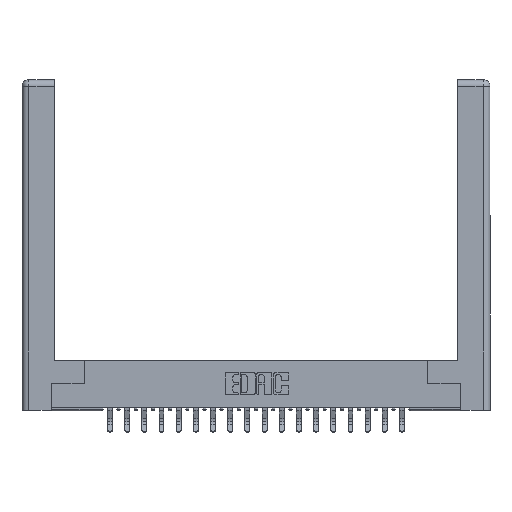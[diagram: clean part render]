
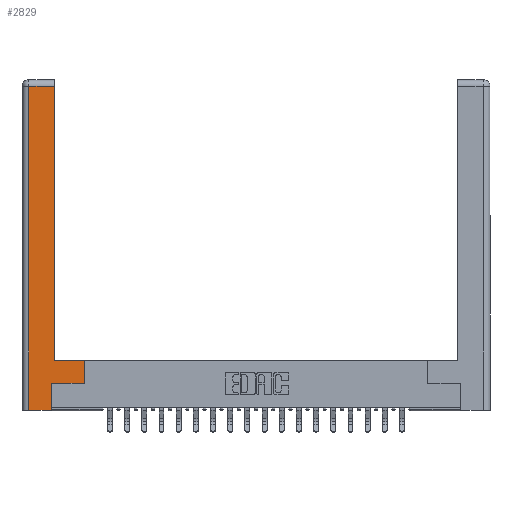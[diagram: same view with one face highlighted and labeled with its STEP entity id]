
A CAD part, top view. The second image highlights one B-rep face of the part: STEP entity #2829.
In plain terms, the highlighted planar face has unit normal (0, 0, 1).
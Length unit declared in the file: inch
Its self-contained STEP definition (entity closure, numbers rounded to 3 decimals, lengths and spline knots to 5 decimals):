
#114 = EDGE_CURVE ( 'NONE', #10199, #15605, #15759, .T. ) ;
#343 = VERTEX_POINT ( 'NONE', #11007 ) ;
#476 = ORIENTED_EDGE ( 'NONE', *, *, #8316, .T. ) ;
#874 = VERTEX_POINT ( 'NONE', #24880 ) ;
#950 = FACE_OUTER_BOUND ( 'NONE', #5604, .T. ) ;
#991 = EDGE_CURVE ( 'NONE', #9284, #343, #18439, .T. ) ;
#1299 = DIRECTION ( 'NONE',  ( 0., 0., -1. ) ) ;
#1379 = CARTESIAN_POINT ( 'NONE',  ( 0., 0., 0. ) ) ;
#2542 = VECTOR ( 'NONE', #3873, 39.37008 ) ;
#2829 = ADVANCED_FACE ( 'NONE', ( #950 ), #22866, .F. ) ;
#3343 = CARTESIAN_POINT ( 'NONE',  ( 0.0615, 2.94, 0. ) ) ;
#3873 = DIRECTION ( 'NONE',  ( 0., 1., 0. ) ) ;
#4245 = DIRECTION ( 'NONE',  ( -1., 0., 0. ) ) ;
#4337 = VECTOR ( 'NONE', #21157, 39.37008 ) ;
#5604 = EDGE_LOOP ( 'NONE', ( #15982, #12240, #10795, #15543, #21265, #24554, #12148, #476 ) ) ;
#5659 = CARTESIAN_POINT ( 'NONE',  ( 0.265, 0., 0. ) ) ;
#5942 = EDGE_CURVE ( 'NONE', #15605, #12000, #15135, .T. ) ;
#6504 = DIRECTION ( 'NONE',  ( 0., -1., 0. ) ) ;
#6518 = EDGE_CURVE ( 'NONE', #7420, #9284, #14197, .T. ) ;
#6595 = LINE ( 'NONE', #22156, #20890 ) ;
#6695 = AXIS2_PLACEMENT_3D ( 'NONE', #1379, #1299, #22707 ) ;
#6805 = CARTESIAN_POINT ( 'NONE',  ( 0.565, 0.245, 0. ) ) ;
#7385 = LINE ( 'NONE', #15557, #4337 ) ;
#7420 = VERTEX_POINT ( 'NONE', #15808 ) ;
#7740 = LINE ( 'NONE', #23475, #2542 ) ;
#8316 = EDGE_CURVE ( 'NONE', #343, #10199, #7385, .T. ) ;
#8689 = DIRECTION ( 'NONE',  ( 1., 0., 0. ) ) ;
#9004 = VECTOR ( 'NONE', #17351, 39.37008 ) ;
#9284 = VERTEX_POINT ( 'NONE', #11108 ) ;
#9619 = CARTESIAN_POINT ( 'NONE',  ( 0.565, 0.45, 0. ) ) ;
#9972 = VECTOR ( 'NONE', #4245, 39.37008 ) ;
#10199 = VERTEX_POINT ( 'NONE', #23012 ) ;
#10268 = CARTESIAN_POINT ( 'NONE',  ( 0.295, 3., 0. ) ) ;
#10795 = ORIENTED_EDGE ( 'NONE', *, *, #22169, .T. ) ;
#11007 = CARTESIAN_POINT ( 'NONE',  ( 0.565, 0.45, 0. ) ) ;
#11108 = CARTESIAN_POINT ( 'NONE',  ( 0.565, 0.245, 0. ) ) ;
#12000 = VERTEX_POINT ( 'NONE', #3343 ) ;
#12148 = ORIENTED_EDGE ( 'NONE', *, *, #991, .T. ) ;
#12240 = ORIENTED_EDGE ( 'NONE', *, *, #5942, .T. ) ;
#12391 = VECTOR ( 'NONE', #22074, 39.37008 ) ;
#12485 = EDGE_CURVE ( 'NONE', #22532, #874, #14129, .T. ) ;
#13222 = DIRECTION ( 'NONE',  ( 1., 0., 0. ) ) ;
#13945 = CARTESIAN_POINT ( 'NONE',  ( 0.0615, 2.94, 0. ) ) ;
#14129 = LINE ( 'NONE', #5659, #19903 ) ;
#14197 = LINE ( 'NONE', #6805, #16659 ) ;
#14323 = CARTESIAN_POINT ( 'NONE',  ( 0.0615, 0., 0. ) ) ;
#15135 = LINE ( 'NONE', #13945, #9972 ) ;
#15543 = ORIENTED_EDGE ( 'NONE', *, *, #12485, .T. ) ;
#15557 = CARTESIAN_POINT ( 'NONE',  ( 0.295, 0.45, 0. ) ) ;
#15605 = VERTEX_POINT ( 'NONE', #23702 ) ;
#15759 = LINE ( 'NONE', #10268, #12391 ) ;
#15808 = CARTESIAN_POINT ( 'NONE',  ( 0.265, 0.245, 0. ) ) ;
#15982 = ORIENTED_EDGE ( 'NONE', *, *, #114, .T. ) ;
#16659 = VECTOR ( 'NONE', #8689, 39.37008 ) ;
#17351 = DIRECTION ( 'NONE',  ( 0., 1., 0. ) ) ;
#18030 = EDGE_CURVE ( 'NONE', #874, #7420, #7740, .T. ) ;
#18439 = LINE ( 'NONE', #9619, #9004 ) ;
#19903 = VECTOR ( 'NONE', #13222, 39.37008 ) ;
#20890 = VECTOR ( 'NONE', #6504, 39.37008 ) ;
#21157 = DIRECTION ( 'NONE',  ( -1., 0., 0. ) ) ;
#21265 = ORIENTED_EDGE ( 'NONE', *, *, #18030, .T. ) ;
#22074 = DIRECTION ( 'NONE',  ( 0., 1., 0. ) ) ;
#22156 = CARTESIAN_POINT ( 'NONE',  ( 0.0615, 0., 0. ) ) ;
#22169 = EDGE_CURVE ( 'NONE', #12000, #22532, #6595, .T. ) ;
#22532 = VERTEX_POINT ( 'NONE', #14323 ) ;
#22707 = DIRECTION ( 'NONE',  ( -1., 0., 0. ) ) ;
#22866 = PLANE ( 'NONE',  #6695 ) ;
#23012 = CARTESIAN_POINT ( 'NONE',  ( 0.295, 0.45, 0. ) ) ;
#23475 = CARTESIAN_POINT ( 'NONE',  ( 0.265, 0.245, 0. ) ) ;
#23702 = CARTESIAN_POINT ( 'NONE',  ( 0.295, 2.94, 0. ) ) ;
#24554 = ORIENTED_EDGE ( 'NONE', *, *, #6518, .T. ) ;
#24880 = CARTESIAN_POINT ( 'NONE',  ( 0.265, 0., 0. ) ) ;
